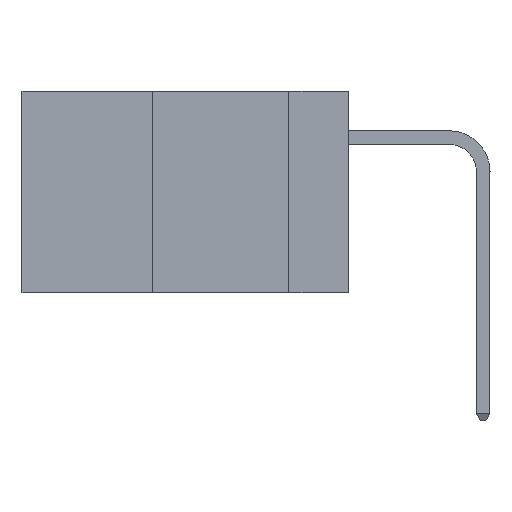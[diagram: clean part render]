
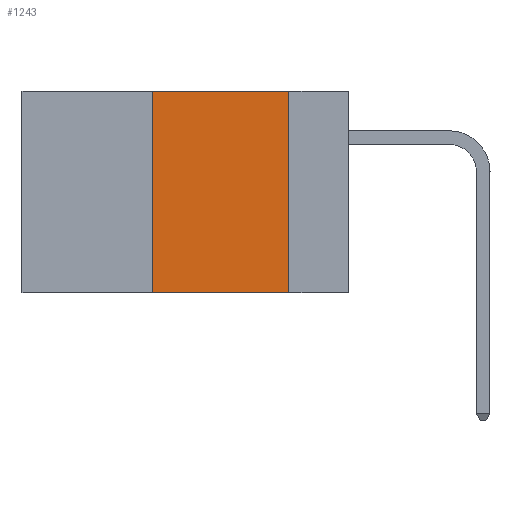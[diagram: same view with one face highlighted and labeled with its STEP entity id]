
A CAD part, left-side view. The second image highlights one B-rep face of the part: STEP entity #1243.
In plain terms, the highlighted planar face has unit normal (-1, 0, 0).
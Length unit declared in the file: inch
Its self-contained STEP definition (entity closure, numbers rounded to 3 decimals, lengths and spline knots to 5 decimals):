
#1243 = ADVANCED_FACE ( 'NONE', ( #11287 ), #8819, .F. ) ;
#1688 = ORIENTED_EDGE ( 'NONE', *, *, #12228, .T. ) ;
#2246 = ORIENTED_EDGE ( 'NONE', *, *, #6962, .F. ) ;
#3064 = VECTOR ( 'NONE', #13652, 39.37008 ) ;
#3604 = LINE ( 'NONE', #11502, #9192 ) ;
#3696 = LINE ( 'NONE', #13625, #7013 ) ;
#3768 = DIRECTION ( 'NONE',  ( 0., -1., 0. ) ) ;
#4287 = VERTEX_POINT ( 'NONE', #7387 ) ;
#4340 = CARTESIAN_POINT ( 'NONE',  ( 0., 0.11, 0. ) ) ;
#4566 = CARTESIAN_POINT ( 'NONE',  ( 0., 0.36, -0.37 ) ) ;
#5512 = VERTEX_POINT ( 'NONE', #4340 ) ;
#5604 = DIRECTION ( 'NONE',  ( 0., 0., -1. ) ) ;
#6264 = VERTEX_POINT ( 'NONE', #4566 ) ;
#6447 = ORIENTED_EDGE ( 'NONE', *, *, #9019, .F. ) ;
#6586 = CARTESIAN_POINT ( 'NONE',  ( 0., 0.36, 0. ) ) ;
#6920 = LINE ( 'NONE', #8203, #12095 ) ;
#6962 = EDGE_CURVE ( 'NONE', #6264, #7347, #6920, .T. ) ;
#6974 = EDGE_CURVE ( 'NONE', #7347, #5512, #3604, .T. ) ;
#7013 = VECTOR ( 'NONE', #8068, 39.37008 ) ;
#7347 = VERTEX_POINT ( 'NONE', #6586 ) ;
#7387 = CARTESIAN_POINT ( 'NONE',  ( 0., 0.11, -0.37 ) ) ;
#7664 = ORIENTED_EDGE ( 'NONE', *, *, #6974, .F. ) ;
#8068 = DIRECTION ( 'NONE',  ( 0., 0., -1. ) ) ;
#8078 = CARTESIAN_POINT ( 'NONE',  ( 0., 0.6, 0. ) ) ;
#8203 = CARTESIAN_POINT ( 'NONE',  ( 0., 0.36, 0. ) ) ;
#8819 = PLANE ( 'NONE',  #12222 ) ;
#9006 = LINE ( 'NONE', #12543, #3064 ) ;
#9019 = EDGE_CURVE ( 'NONE', #5512, #4287, #3696, .T. ) ;
#9192 = VECTOR ( 'NONE', #3768, 39.37008 ) ;
#9330 = DIRECTION ( 'NONE',  ( 0., 0., 1. ) ) ;
#9932 = DIRECTION ( 'NONE',  ( 1., 0., 0. ) ) ;
#11287 = FACE_OUTER_BOUND ( 'NONE', #14031, .T. ) ;
#11502 = CARTESIAN_POINT ( 'NONE',  ( 0., 0.6, 0. ) ) ;
#12095 = VECTOR ( 'NONE', #9330, 39.37008 ) ;
#12222 = AXIS2_PLACEMENT_3D ( 'NONE', #8078, #9932, #5604 ) ;
#12228 = EDGE_CURVE ( 'NONE', #6264, #4287, #9006, .T. ) ;
#12543 = CARTESIAN_POINT ( 'NONE',  ( 0., 0.6, -0.37 ) ) ;
#13625 = CARTESIAN_POINT ( 'NONE',  ( 0., 0.11, 0. ) ) ;
#13652 = DIRECTION ( 'NONE',  ( 0., -1., 0. ) ) ;
#14031 = EDGE_LOOP ( 'NONE', ( #6447, #7664, #2246, #1688 ) ) ;
